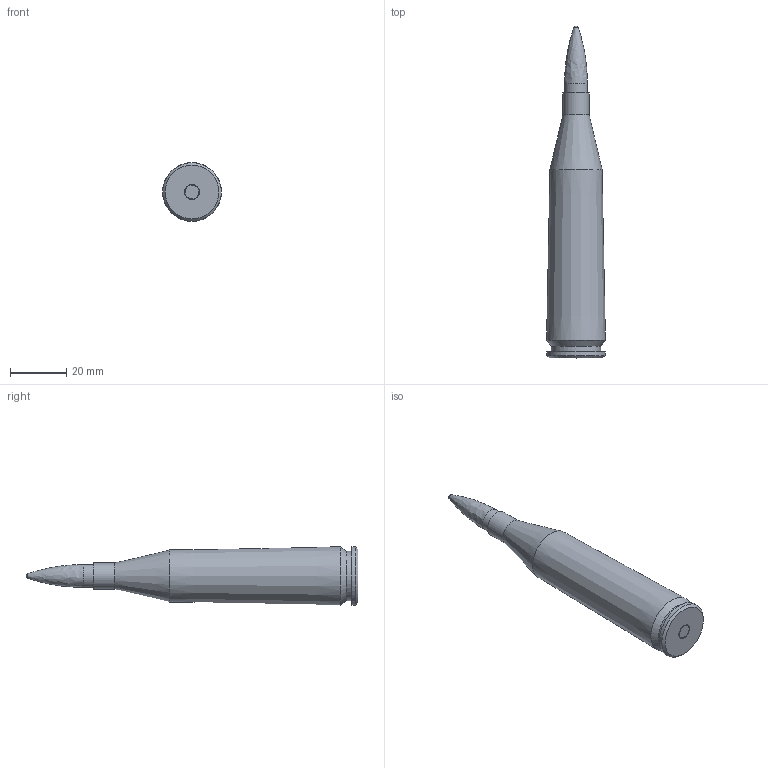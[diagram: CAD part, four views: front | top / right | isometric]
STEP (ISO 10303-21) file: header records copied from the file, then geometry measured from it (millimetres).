
FILE_DESCRIPTION((''),'2;1');
FILE_NAME('7.92X94MM PANZERBUCHSE.stp','2012-12-03T13:10:40',('agarrett'),(''),'Autodesk Inventor 2012','Autodesk Inventor 2012','');
FILE_SCHEMA(('AUTOMOTIVE_DESIGN { 1 0 10303 214 1 1 1 1 }'));
Length unit declared in the file: inch
Products named in the file (4): iLogic Cartridge; Rimless Bottleneck; iLogic SP Bullet; PRIMER
Assembly tree (3 placements, depth 2):
  iLogic Cartridge
    Rimless Bottleneck
    iLogic SP Bullet
    PRIMER
Bounding box: 20.95 x 118.28 x 20.95 mm (x, y, z)
Volume: 5577.3 mm3; surface area: 11785.2 mm2
Topology: 3 solids, 3 shells, 33 faces, 55 edges, 31 vertices
Faces by surface type: cylinder 9, plane 8, cone 7, torus 7, sphere 1, bspline 1
Full cylindrical faces by diameter (mm): 1.778 x1, 5.08 x1, 5.334 x2, 8.204 x2, 9.373 x1, 17.475 x1, 20.879 x1
Entity records: 804 total; most frequent: DIRECTION 140, CARTESIAN_POINT 128, AXIS2_PLACEMENT_3D 70, ORIENTED_EDGE 62, EDGE_LOOP 62, FACE_OUTER_BOUND 33, ADVANCED_FACE 33, VERTEX_POINT 31
